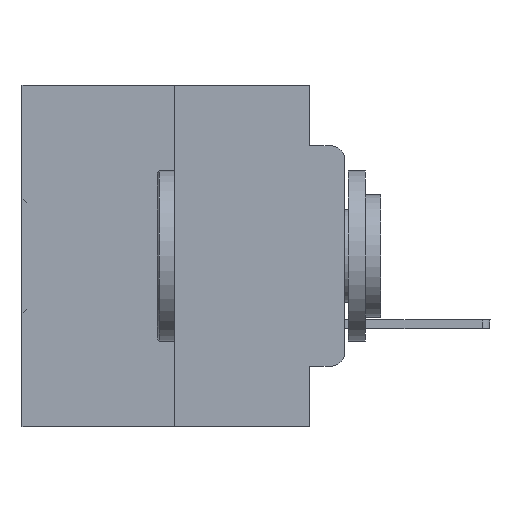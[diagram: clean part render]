
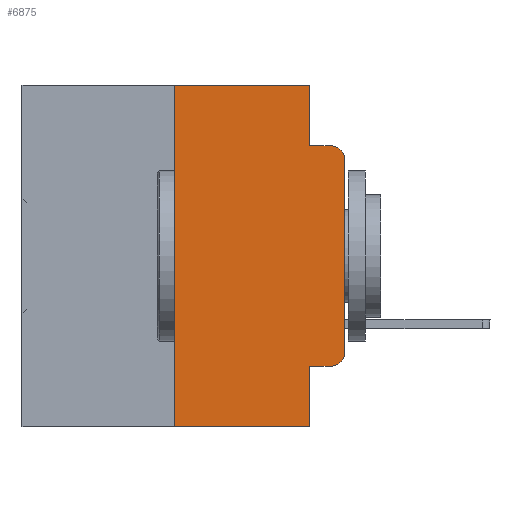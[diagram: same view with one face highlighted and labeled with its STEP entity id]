
A CAD part, left-side view. The second image highlights one B-rep face of the part: STEP entity #6875.
In plain terms, the highlighted planar face has unit normal (-1, 0, 0).
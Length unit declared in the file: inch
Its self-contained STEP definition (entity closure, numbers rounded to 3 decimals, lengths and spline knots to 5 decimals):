
#434 = EDGE_CURVE ( 'NONE', #25400, #27301, #13949, .T. ) ;
#529 = EDGE_CURVE ( 'NONE', #27301, #4732, #15596, .T. ) ;
#721 = CARTESIAN_POINT ( 'NONE',  ( 0., 0.02, -0.4115 ) ) ;
#1683 = LINE ( 'NONE', #27252, #21030 ) ;
#2029 = VECTOR ( 'NONE', #30615, 39.37008 ) ;
#2385 = DIRECTION ( 'NONE',  ( 0., 0., -1. ) ) ;
#2582 = DIRECTION ( 'NONE',  ( 0., 0., -1. ) ) ;
#2800 = CARTESIAN_POINT ( 'NONE',  ( 0., 0.051, 0. ) ) ;
#3280 = CIRCLE ( 'NONE', #32637, 0.02 ) ;
#3431 = ORIENTED_EDGE ( 'NONE', *, *, #434, .F. ) ;
#4240 = VECTOR ( 'NONE', #25790, 39.37008 ) ;
#4411 = EDGE_CURVE ( 'NONE', #4732, #10746, #1683, .T. ) ;
#4732 = VERTEX_POINT ( 'NONE', #18843 ) ;
#4737 = EDGE_CURVE ( 'NONE', #24642, #10746, #3280, .T. ) ;
#5082 = VECTOR ( 'NONE', #9870, 39.37008 ) ;
#6875 = ADVANCED_FACE ( 'NONE', ( #20453 ), #26016, .F. ) ;
#6971 = VECTOR ( 'NONE', #25644, 39.37008 ) ;
#7165 = DIRECTION ( 'NONE',  ( -1., 0., 0. ) ) ;
#7364 = AXIS2_PLACEMENT_3D ( 'NONE', #15547, #10251, #2385 ) ;
#7449 = ORIENTED_EDGE ( 'NONE', *, *, #28456, .F. ) ;
#7694 = DIRECTION ( 'NONE',  ( 0., 0., -1. ) ) ;
#7737 = CARTESIAN_POINT ( 'NONE',  ( 0., 0.25, 0. ) ) ;
#7829 = VERTEX_POINT ( 'NONE', #24030 ) ;
#9834 = CARTESIAN_POINT ( 'NONE',  ( 0., 0.02, -0.0885 ) ) ;
#9870 = DIRECTION ( 'NONE',  ( 0., -1., 0. ) ) ;
#9995 = CARTESIAN_POINT ( 'NONE',  ( 0., 0.473, 0. ) ) ;
#10251 = DIRECTION ( 'NONE',  ( 1., 0., 0. ) ) ;
#10746 = VERTEX_POINT ( 'NONE', #9834 ) ;
#10754 = VERTEX_POINT ( 'NONE', #28246 ) ;
#11214 = LINE ( 'NONE', #28199, #4240 ) ;
#12045 = VERTEX_POINT ( 'NONE', #17012 ) ;
#12088 = LINE ( 'NONE', #33679, #5082 ) ;
#13667 = CARTESIAN_POINT ( 'NONE',  ( 0., 0.02, -0.1085 ) ) ;
#13949 = LINE ( 'NONE', #9995, #6971 ) ;
#13952 = AXIS2_PLACEMENT_3D ( 'NONE', #14348, #7165, #7694 ) ;
#14348 = CARTESIAN_POINT ( 'NONE',  ( 0., 0.02, -0.3915 ) ) ;
#15547 = CARTESIAN_POINT ( 'NONE',  ( 0., 0.473, 0. ) ) ;
#15596 = LINE ( 'NONE', #2800, #22597 ) ;
#15889 = EDGE_CURVE ( 'NONE', #23512, #12045, #25027, .T. ) ;
#15968 = DIRECTION ( 'NONE',  ( 0., 0., -1. ) ) ;
#16013 = ORIENTED_EDGE ( 'NONE', *, *, #4411, .F. ) ;
#16022 = ORIENTED_EDGE ( 'NONE', *, *, #4737, .T. ) ;
#16572 = CARTESIAN_POINT ( 'NONE',  ( 0., 0.473, -0.5 ) ) ;
#17012 = CARTESIAN_POINT ( 'NONE',  ( 0., 0., -0.3915 ) ) ;
#17546 = CARTESIAN_POINT ( 'NONE',  ( 0., 0.051, 0. ) ) ;
#17661 = EDGE_CURVE ( 'NONE', #7829, #25400, #27567, .T. ) ;
#17980 = ORIENTED_EDGE ( 'NONE', *, *, #17661, .F. ) ;
#18222 = EDGE_CURVE ( 'NONE', #7829, #10754, #25066, .T. ) ;
#18395 = ORIENTED_EDGE ( 'NONE', *, *, #24891, .T. ) ;
#18843 = CARTESIAN_POINT ( 'NONE',  ( 0., 0.051, -0.0885 ) ) ;
#18932 = VERTEX_POINT ( 'NONE', #26341 ) ;
#19193 = ORIENTED_EDGE ( 'NONE', *, *, #18222, .T. ) ;
#20124 = LINE ( 'NONE', #20234, #2029 ) ;
#20234 = CARTESIAN_POINT ( 'NONE',  ( 0., 0.051, 0. ) ) ;
#20453 = FACE_OUTER_BOUND ( 'NONE', #26901, .T. ) ;
#20533 = VECTOR ( 'NONE', #26148, 39.37008 ) ;
#21030 = VECTOR ( 'NONE', #22324, 39.37008 ) ;
#22324 = DIRECTION ( 'NONE',  ( 0., -1., 0. ) ) ;
#22597 = VECTOR ( 'NONE', #2582, 39.37008 ) ;
#23512 = VERTEX_POINT ( 'NONE', #721 ) ;
#24030 = CARTESIAN_POINT ( 'NONE',  ( 0., 0.25, -0.5 ) ) ;
#24642 = VERTEX_POINT ( 'NONE', #28597 ) ;
#24891 = EDGE_CURVE ( 'NONE', #12045, #24642, #11214, .T. ) ;
#25027 = CIRCLE ( 'NONE', #13952, 0.02 ) ;
#25066 = LINE ( 'NONE', #16572, #34084 ) ;
#25400 = VERTEX_POINT ( 'NONE', #29645 ) ;
#25609 = EDGE_CURVE ( 'NONE', #18932, #23512, #12088, .T. ) ;
#25644 = DIRECTION ( 'NONE',  ( 0., -1., 0. ) ) ;
#25790 = DIRECTION ( 'NONE',  ( 0., 0., 1. ) ) ;
#26016 = PLANE ( 'NONE',  #7364 ) ;
#26148 = DIRECTION ( 'NONE',  ( 0., 0., 1. ) ) ;
#26341 = CARTESIAN_POINT ( 'NONE',  ( 0., 0.051, -0.4115 ) ) ;
#26901 = EDGE_LOOP ( 'NONE', ( #18395, #16022, #16013, #31930, #3431, #17980, #19193, #7449, #28205, #32879 ) ) ;
#26962 = DIRECTION ( 'NONE',  ( 0., -1., 0. ) ) ;
#27252 = CARTESIAN_POINT ( 'NONE',  ( 0., 0.051, -0.0885 ) ) ;
#27301 = VERTEX_POINT ( 'NONE', #17546 ) ;
#27567 = LINE ( 'NONE', #7737, #20533 ) ;
#28199 = CARTESIAN_POINT ( 'NONE',  ( 0., 0., 0. ) ) ;
#28205 = ORIENTED_EDGE ( 'NONE', *, *, #25609, .T. ) ;
#28246 = CARTESIAN_POINT ( 'NONE',  ( 0., 0.051, -0.5 ) ) ;
#28456 = EDGE_CURVE ( 'NONE', #18932, #10754, #20124, .T. ) ;
#28597 = CARTESIAN_POINT ( 'NONE',  ( 0., 0., -0.1085 ) ) ;
#29201 = DIRECTION ( 'NONE',  ( -1., 0., 0. ) ) ;
#29645 = CARTESIAN_POINT ( 'NONE',  ( 0., 0.25, 0. ) ) ;
#30615 = DIRECTION ( 'NONE',  ( 0., 0., -1. ) ) ;
#31930 = ORIENTED_EDGE ( 'NONE', *, *, #529, .F. ) ;
#32637 = AXIS2_PLACEMENT_3D ( 'NONE', #13667, #29201, #15968 ) ;
#32879 = ORIENTED_EDGE ( 'NONE', *, *, #15889, .T. ) ;
#33679 = CARTESIAN_POINT ( 'NONE',  ( 0., 0.051, -0.4115 ) ) ;
#34084 = VECTOR ( 'NONE', #26962, 39.37008 ) ;
